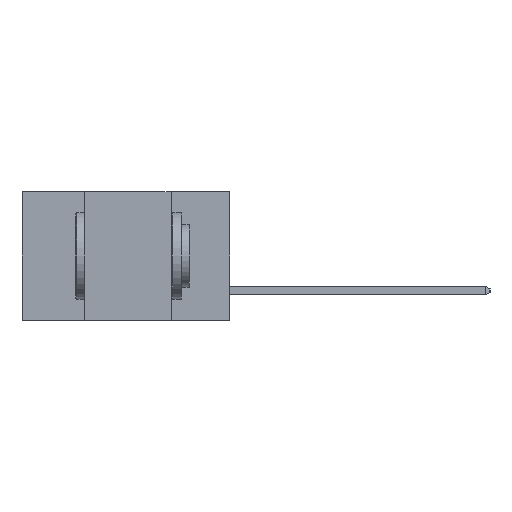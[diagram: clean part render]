
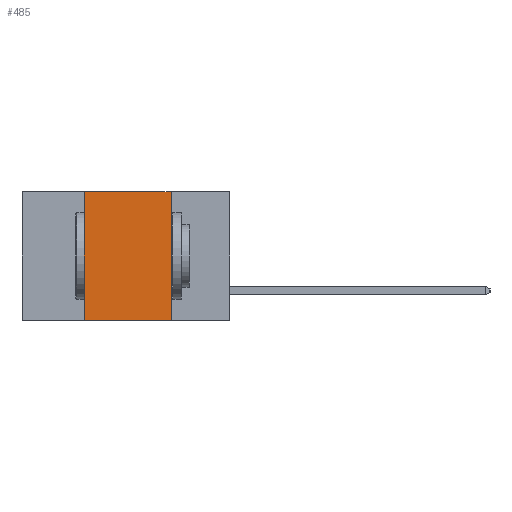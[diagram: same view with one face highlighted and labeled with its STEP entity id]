
A CAD part, left-side view. The second image highlights one B-rep face of the part: STEP entity #485.
In plain terms, the highlighted planar face has unit normal (-1, 0, 0).
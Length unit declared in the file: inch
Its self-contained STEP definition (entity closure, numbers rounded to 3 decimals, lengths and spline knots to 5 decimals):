
#79 = VECTOR ( 'NONE', #6659, 39.37008 ) ;
#472 = VERTEX_POINT ( 'NONE', #1280 ) ;
#485 = ADVANCED_FACE ( 'NONE', ( #2596 ), #518, .F. ) ;
#518 = PLANE ( 'NONE',  #4733 ) ;
#543 = ORIENTED_EDGE ( 'NONE', *, *, #1951, .F. ) ;
#713 = EDGE_LOOP ( 'NONE', ( #1840, #543, #3634, #4709 ) ) ;
#1280 = CARTESIAN_POINT ( 'NONE',  ( 0., 0.17, 0. ) ) ;
#1428 = CARTESIAN_POINT ( 'NONE',  ( 0., 0.42, -0.37 ) ) ;
#1840 = ORIENTED_EDGE ( 'NONE', *, *, #8127, .F. ) ;
#1951 = EDGE_CURVE ( 'NONE', #3896, #472, #6488, .T. ) ;
#1984 = LINE ( 'NONE', #1428, #9129 ) ;
#2492 = VECTOR ( 'NONE', #5549, 39.37008 ) ;
#2578 = VERTEX_POINT ( 'NONE', #7870 ) ;
#2596 = FACE_OUTER_BOUND ( 'NONE', #713, .T. ) ;
#2845 = DIRECTION ( 'NONE',  ( 1., 0., 0. ) ) ;
#3163 = VERTEX_POINT ( 'NONE', #9102 ) ;
#3595 = EDGE_CURVE ( 'NONE', #3163, #2578, #5923, .T. ) ;
#3611 = DIRECTION ( 'NONE',  ( 0., 0., 1. ) ) ;
#3626 = DIRECTION ( 'NONE',  ( 0., 0., -1. ) ) ;
#3634 = ORIENTED_EDGE ( 'NONE', *, *, #7365, .F. ) ;
#3753 = CARTESIAN_POINT ( 'NONE',  ( 0., 0.6, 0. ) ) ;
#3896 = VERTEX_POINT ( 'NONE', #5159 ) ;
#4574 = CARTESIAN_POINT ( 'NONE',  ( 0., 0.6, 0. ) ) ;
#4709 = ORIENTED_EDGE ( 'NONE', *, *, #3595, .T. ) ;
#4733 = AXIS2_PLACEMENT_3D ( 'NONE', #4574, #2845, #3626 ) ;
#5159 = CARTESIAN_POINT ( 'NONE',  ( 0., 0.42, 0. ) ) ;
#5549 = DIRECTION ( 'NONE',  ( 0., -1., 0. ) ) ;
#5923 = LINE ( 'NONE', #6668, #79 ) ;
#6488 = LINE ( 'NONE', #3753, #2492 ) ;
#6513 = DIRECTION ( 'NONE',  ( 0., 0., -1. ) ) ;
#6659 = DIRECTION ( 'NONE',  ( 0., -1., 0. ) ) ;
#6662 = VECTOR ( 'NONE', #6513, 39.37008 ) ;
#6668 = CARTESIAN_POINT ( 'NONE',  ( 0., 0.6, -0.37 ) ) ;
#7175 = CARTESIAN_POINT ( 'NONE',  ( 0., 0.17, -0.37 ) ) ;
#7365 = EDGE_CURVE ( 'NONE', #3163, #3896, #1984, .T. ) ;
#7870 = CARTESIAN_POINT ( 'NONE',  ( 0., 0.17, -0.37 ) ) ;
#8127 = EDGE_CURVE ( 'NONE', #472, #2578, #8478, .T. ) ;
#8478 = LINE ( 'NONE', #7175, #6662 ) ;
#9102 = CARTESIAN_POINT ( 'NONE',  ( 0., 0.42, -0.37 ) ) ;
#9129 = VECTOR ( 'NONE', #3611, 39.37008 ) ;
